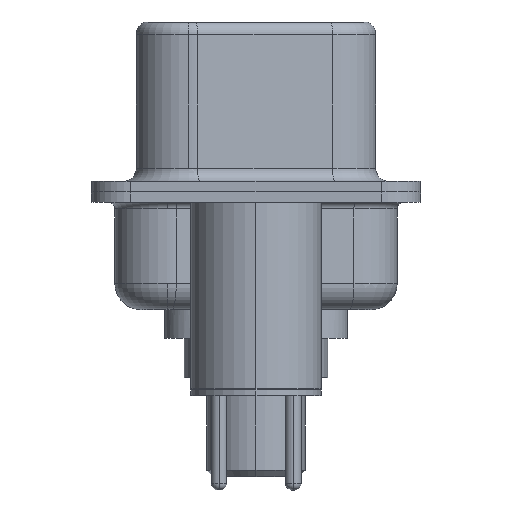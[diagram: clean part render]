
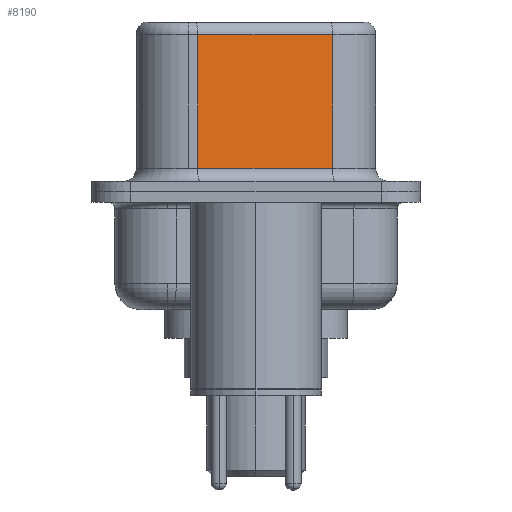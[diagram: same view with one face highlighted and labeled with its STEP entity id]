
A CAD part, left-side view. The second image highlights one B-rep face of the part: STEP entity #8190.
In plain terms, the highlighted planar face has unit normal (-0.985, -0.174, 0).
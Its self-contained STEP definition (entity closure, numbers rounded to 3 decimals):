
#697 = DIRECTION ( 'NONE',  ( -0.174, 0.985, 0. ) ) ;
#2026 = VERTEX_POINT ( 'NONE', #15417 ) ;
#3238 = ORIENTED_EDGE ( 'NONE', *, *, #12113, .F. ) ;
#4418 = CARTESIAN_POINT ( 'NONE',  ( 3.655, 2.233, 6.52 ) ) ;
#4676 = PLANE ( 'NONE',  #9873 ) ;
#5471 = VERTEX_POINT ( 'NONE', #15563 ) ;
#5999 = DIRECTION ( 'NONE',  ( 0.174, -0.985, 0. ) ) ;
#6012 = CARTESIAN_POINT ( 'NONE',  ( 4.565, -2.927, 6.52 ) ) ;
#6016 = ORIENTED_EDGE ( 'NONE', *, *, #13494, .T. ) ;
#8045 = CARTESIAN_POINT ( 'NONE',  ( 3.655, 2.233, 6.02 ) ) ;
#8190 = ADVANCED_FACE ( 'NONE', ( #8897 ), #4676, .F. ) ;
#8737 = EDGE_CURVE ( 'NONE', #10528, #15319, #10932, .T. ) ;
#8897 = FACE_OUTER_BOUND ( 'NONE', #14588, .T. ) ;
#8944 = LINE ( 'NONE', #17049, #15817 ) ;
#9873 = AXIS2_PLACEMENT_3D ( 'NONE', #6012, #11531, #15619 ) ;
#10059 = DIRECTION ( 'NONE',  ( 0., 0., -1. ) ) ;
#10178 = CARTESIAN_POINT ( 'NONE',  ( 4.565, -2.927, 0.9 ) ) ;
#10340 = VECTOR ( 'NONE', #5999, 1000. ) ;
#10528 = VERTEX_POINT ( 'NONE', #8045 ) ;
#10932 = LINE ( 'NONE', #4418, #16793 ) ;
#11023 = ORIENTED_EDGE ( 'NONE', *, *, #8737, .T. ) ;
#11227 = VECTOR ( 'NONE', #10059, 1000. ) ;
#11531 = DIRECTION ( 'NONE',  ( 0.985, 0.174, 0. ) ) ;
#11643 = LINE ( 'NONE', #14163, #11227 ) ;
#12113 = EDGE_CURVE ( 'NONE', #2026, #5471, #11643, .T. ) ;
#12138 = EDGE_CURVE ( 'NONE', #15319, #5471, #14016, .T. ) ;
#12528 = ORIENTED_EDGE ( 'NONE', *, *, #12138, .T. ) ;
#13494 = EDGE_CURVE ( 'NONE', #2026, #10528, #8944, .T. ) ;
#14016 = LINE ( 'NONE', #10178, #10340 ) ;
#14037 = DIRECTION ( 'NONE',  ( 0., 0., -1. ) ) ;
#14163 = CARTESIAN_POINT ( 'NONE',  ( 4.565, -2.927, 6.52 ) ) ;
#14588 = EDGE_LOOP ( 'NONE', ( #3238, #6016, #11023, #12528 ) ) ;
#15319 = VERTEX_POINT ( 'NONE', #16654 ) ;
#15417 = CARTESIAN_POINT ( 'NONE',  ( 4.565, -2.927, 6.02 ) ) ;
#15563 = CARTESIAN_POINT ( 'NONE',  ( 4.565, -2.927, 0.9 ) ) ;
#15619 = DIRECTION ( 'NONE',  ( -0.174, 0.985, 0. ) ) ;
#15817 = VECTOR ( 'NONE', #697, 1000. ) ;
#16654 = CARTESIAN_POINT ( 'NONE',  ( 3.655, 2.233, 0.9 ) ) ;
#16793 = VECTOR ( 'NONE', #14037, 1000. ) ;
#17049 = CARTESIAN_POINT ( 'NONE',  ( 4.565, -2.927, 6.02 ) ) ;
